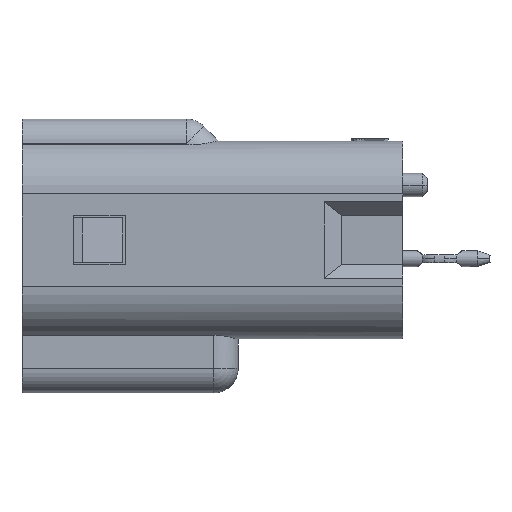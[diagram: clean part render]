
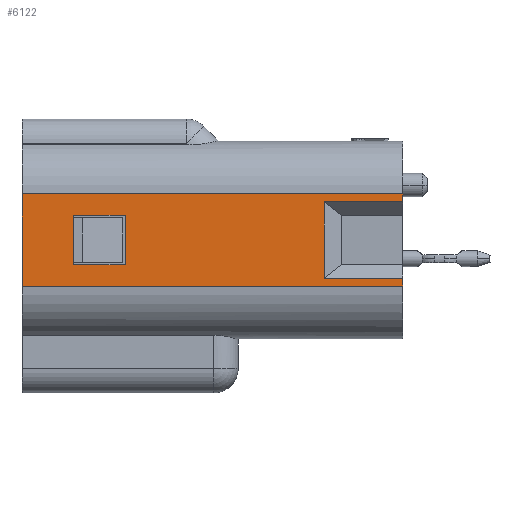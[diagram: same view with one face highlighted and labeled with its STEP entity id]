
A CAD part, left-side view. The second image highlights one B-rep face of the part: STEP entity #6122.
In plain terms, the highlighted planar face has unit normal (-1, 0, 0).
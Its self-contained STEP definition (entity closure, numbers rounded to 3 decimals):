
#256 = LINE ( 'NONE', #12996, #2669 ) ;
#702 = ORIENTED_EDGE ( 'NONE', *, *, #2418, .T. ) ;
#852 = DIRECTION ( 'NONE',  ( 0., 0., 1. ) ) ;
#896 = ORIENTED_EDGE ( 'NONE', *, *, #5673, .T. ) ;
#946 = VECTOR ( 'NONE', #852, 1000. ) ;
#1519 = DIRECTION ( 'NONE',  ( 0., -1., 0. ) ) ;
#1699 = EDGE_LOOP ( 'NONE', ( #16178, #16468, #9885, #702 ) ) ;
#1922 = CARTESIAN_POINT ( 'NONE',  ( 0., 5.225, -16.95 ) ) ;
#1934 = EDGE_CURVE ( 'NONE', #17758, #11366, #13842, .T. ) ;
#1980 = EDGE_CURVE ( 'NONE', #7305, #15628, #16889, .T. ) ;
#2095 = VECTOR ( 'NONE', #4126, 1000. ) ;
#2123 = DIRECTION ( 'NONE',  ( 0., -1., 0. ) ) ;
#2418 = EDGE_CURVE ( 'NONE', #16852, #17758, #15216, .T. ) ;
#2566 = DIRECTION ( 'NONE',  ( 0., -1., 0. ) ) ;
#2575 = CARTESIAN_POINT ( 'NONE',  ( 0., 8.1, -19.05 ) ) ;
#2669 = VECTOR ( 'NONE', #17243, 1000. ) ;
#2730 = ORIENTED_EDGE ( 'NONE', *, *, #3772, .T. ) ;
#2786 = CARTESIAN_POINT ( 'NONE',  ( 0., 5.225, -14.85 ) ) ;
#2843 = EDGE_CURVE ( 'NONE', #11366, #12604, #6669, .T. ) ;
#2896 = CARTESIAN_POINT ( 'NONE',  ( 0., 4.35, -3.55 ) ) ;
#3260 = CARTESIAN_POINT ( 'NONE',  ( 0., 5.225, -14.85 ) ) ;
#3536 = ORIENTED_EDGE ( 'NONE', *, *, #15875, .F. ) ;
#3602 = DIRECTION ( 'NONE',  ( -1., 0., 0. ) ) ;
#3670 = VERTEX_POINT ( 'NONE', #17972 ) ;
#3772 = EDGE_CURVE ( 'NONE', #7305, #6679, #5582, .T. ) ;
#3789 = CARTESIAN_POINT ( 'NONE',  ( 0., 4.675, -6.75 ) ) ;
#4037 = CARTESIAN_POINT ( 'NONE',  ( 0., 8.1, -19.05 ) ) ;
#4126 = DIRECTION ( 'NONE',  ( 0., -1., 0. ) ) ;
#4271 = LINE ( 'NONE', #7129, #17639 ) ;
#4359 = CARTESIAN_POINT ( 'NONE',  ( 0., 4.35, -19.05 ) ) ;
#4465 = CARTESIAN_POINT ( 'NONE',  ( 0., 8.1, -19.05 ) ) ;
#4694 = VECTOR ( 'NONE', #15483, 1000. ) ;
#5506 = ORIENTED_EDGE ( 'NONE', *, *, #15958, .F. ) ;
#5582 = LINE ( 'NONE', #4465, #18220 ) ;
#5673 = EDGE_CURVE ( 'NONE', #16950, #3670, #9427, .T. ) ;
#5763 = CARTESIAN_POINT ( 'NONE',  ( 0., 4.675, -3.55 ) ) ;
#6090 = ORIENTED_EDGE ( 'NONE', *, *, #12695, .T. ) ;
#6122 = ADVANCED_FACE ( 'NONE', ( #10608, #15062 ), #6730, .T. ) ;
#6163 = LINE ( 'NONE', #1922, #6314 ) ;
#6293 = VECTOR ( 'NONE', #2123, 1000. ) ;
#6314 = VECTOR ( 'NONE', #8651, 1000. ) ;
#6444 = LINE ( 'NONE', #12091, #6293 ) ;
#6474 = CARTESIAN_POINT ( 'NONE',  ( 0., 7.775, -6.75 ) ) ;
#6669 = LINE ( 'NONE', #2786, #9398 ) ;
#6679 = VERTEX_POINT ( 'NONE', #4359 ) ;
#6730 = PLANE ( 'NONE',  #16099 ) ;
#7129 = CARTESIAN_POINT ( 'NONE',  ( 0., 4.35, -19.05 ) ) ;
#7305 = VERTEX_POINT ( 'NONE', #16364 ) ;
#7332 = ORIENTED_EDGE ( 'NONE', *, *, #1980, .F. ) ;
#7699 = EDGE_CURVE ( 'NONE', #12604, #16852, #6163, .T. ) ;
#8104 = CARTESIAN_POINT ( 'NONE',  ( 0., 8.1, -3.55 ) ) ;
#8509 = EDGE_CURVE ( 'NONE', #6679, #12857, #4271, .T. ) ;
#8651 = DIRECTION ( 'NONE',  ( 0., 1., 0. ) ) ;
#8845 = CARTESIAN_POINT ( 'NONE',  ( 0., 8.1, -3.55 ) ) ;
#9398 = VECTOR ( 'NONE', #16933, 1000. ) ;
#9427 = LINE ( 'NONE', #6474, #946 ) ;
#9586 = LINE ( 'NONE', #8104, #13109 ) ;
#9732 = CARTESIAN_POINT ( 'NONE',  ( 0., 7.225, -16.95 ) ) ;
#9783 = LINE ( 'NONE', #3789, #13670 ) ;
#9885 = ORIENTED_EDGE ( 'NONE', *, *, #7699, .T. ) ;
#10608 = FACE_BOUND ( 'NONE', #1699, .T. ) ;
#10938 = CARTESIAN_POINT ( 'NONE',  ( 0., 4.675, -6.75 ) ) ;
#10991 = DIRECTION ( 'NONE',  ( 0., 1., 0. ) ) ;
#11364 = CARTESIAN_POINT ( 'NONE',  ( 0., 7.775, -6.75 ) ) ;
#11366 = VERTEX_POINT ( 'NONE', #3260 ) ;
#12091 = CARTESIAN_POINT ( 'NONE',  ( 0., 4.675, -3.55 ) ) ;
#12188 = DIRECTION ( 'NONE',  ( 0., -1., 0. ) ) ;
#12604 = VERTEX_POINT ( 'NONE', #14473 ) ;
#12695 = EDGE_CURVE ( 'NONE', #14171, #13995, #256, .T. ) ;
#12857 = VERTEX_POINT ( 'NONE', #2896 ) ;
#12996 = CARTESIAN_POINT ( 'NONE',  ( 0., 4.675, -3.55 ) ) ;
#13109 = VECTOR ( 'NONE', #2566, 1000. ) ;
#13670 = VECTOR ( 'NONE', #10991, 1000. ) ;
#13842 = LINE ( 'NONE', #13933, #2095 ) ;
#13896 = VECTOR ( 'NONE', #15597, 1000. ) ;
#13933 = CARTESIAN_POINT ( 'NONE',  ( 0., 7.225, -14.85 ) ) ;
#13995 = VERTEX_POINT ( 'NONE', #10938 ) ;
#14104 = ORIENTED_EDGE ( 'NONE', *, *, #15533, .T. ) ;
#14171 = VERTEX_POINT ( 'NONE', #5763 ) ;
#14274 = CARTESIAN_POINT ( 'NONE',  ( 0., 7.225, -14.85 ) ) ;
#14473 = CARTESIAN_POINT ( 'NONE',  ( 0., 5.225, -16.95 ) ) ;
#15062 = FACE_OUTER_BOUND ( 'NONE', #16830, .T. ) ;
#15216 = LINE ( 'NONE', #9732, #4694 ) ;
#15483 = DIRECTION ( 'NONE',  ( 0., 0., 1. ) ) ;
#15533 = EDGE_CURVE ( 'NONE', #13995, #16950, #9783, .T. ) ;
#15597 = DIRECTION ( 'NONE',  ( 0., 0., 1. ) ) ;
#15628 = VERTEX_POINT ( 'NONE', #8845 ) ;
#15837 = DIRECTION ( 'NONE',  ( 0., 0., 1. ) ) ;
#15875 = EDGE_CURVE ( 'NONE', #14171, #12857, #6444, .T. ) ;
#15958 = EDGE_CURVE ( 'NONE', #15628, #3670, #9586, .T. ) ;
#16099 = AXIS2_PLACEMENT_3D ( 'NONE', #2575, #3602, #12188 ) ;
#16178 = ORIENTED_EDGE ( 'NONE', *, *, #1934, .T. ) ;
#16364 = CARTESIAN_POINT ( 'NONE',  ( 0., 8.1, -19.05 ) ) ;
#16468 = ORIENTED_EDGE ( 'NONE', *, *, #2843, .T. ) ;
#16578 = ORIENTED_EDGE ( 'NONE', *, *, #8509, .T. ) ;
#16830 = EDGE_LOOP ( 'NONE', ( #896, #5506, #7332, #2730, #16578, #3536, #6090, #14104 ) ) ;
#16852 = VERTEX_POINT ( 'NONE', #18121 ) ;
#16889 = LINE ( 'NONE', #4037, #13896 ) ;
#16933 = DIRECTION ( 'NONE',  ( 0., 0., -1. ) ) ;
#16950 = VERTEX_POINT ( 'NONE', #11364 ) ;
#17243 = DIRECTION ( 'NONE',  ( 0., 0., -1. ) ) ;
#17639 = VECTOR ( 'NONE', #15837, 1000. ) ;
#17758 = VERTEX_POINT ( 'NONE', #14274 ) ;
#17972 = CARTESIAN_POINT ( 'NONE',  ( 0., 7.775, -3.55 ) ) ;
#18121 = CARTESIAN_POINT ( 'NONE',  ( 0., 7.225, -16.95 ) ) ;
#18220 = VECTOR ( 'NONE', #1519, 1000. ) ;
